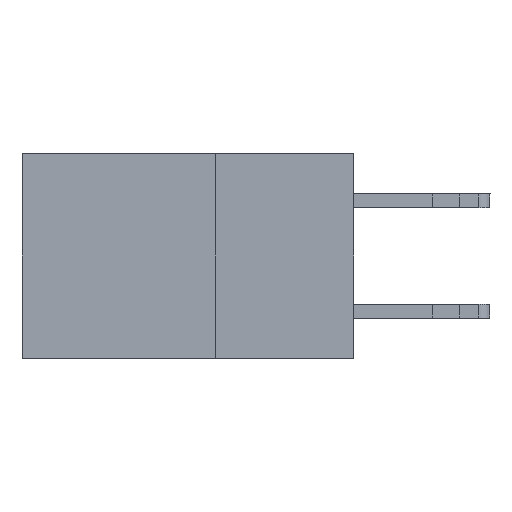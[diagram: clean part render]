
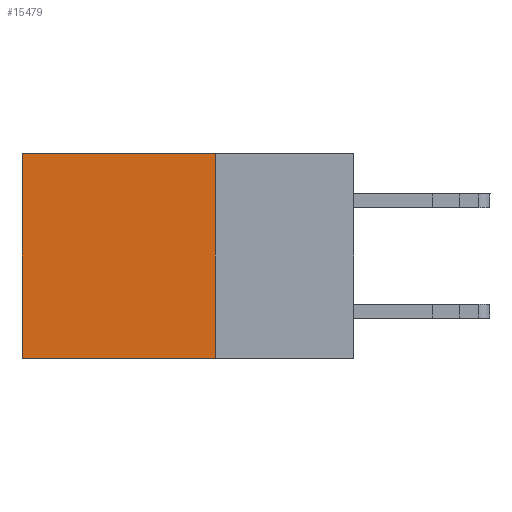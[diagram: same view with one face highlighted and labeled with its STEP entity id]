
A CAD part, left-side view. The second image highlights one B-rep face of the part: STEP entity #15479.
In plain terms, the highlighted planar face has unit normal (-1, 0, 0).
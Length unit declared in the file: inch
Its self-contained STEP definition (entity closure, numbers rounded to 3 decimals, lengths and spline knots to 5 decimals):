
#944 = FACE_OUTER_BOUND ( 'NONE', #14228, .T. ) ;
#1992 = VECTOR ( 'NONE', #2763, 39.37008 ) ;
#2371 = VERTEX_POINT ( 'NONE', #12612 ) ;
#2507 = CARTESIAN_POINT ( 'NONE',  ( 0.2875, 0.25, 0. ) ) ;
#2763 = DIRECTION ( 'NONE',  ( 0., 1., 0. ) ) ;
#3121 = CARTESIAN_POINT ( 'NONE',  ( 0.2875, 0.6, -0.37 ) ) ;
#3181 = VERTEX_POINT ( 'NONE', #2507 ) ;
#4459 = CARTESIAN_POINT ( 'NONE',  ( 0.2875, 0.25, 0. ) ) ;
#5456 = LINE ( 'NONE', #13722, #12056 ) ;
#5554 = LINE ( 'NONE', #9321, #1992 ) ;
#5643 = VERTEX_POINT ( 'NONE', #3121 ) ;
#5786 = DIRECTION ( 'NONE',  ( 0., 1., 0. ) ) ;
#6317 = LINE ( 'NONE', #4459, #16879 ) ;
#6527 = CARTESIAN_POINT ( 'NONE',  ( 0.2875, 0.6, 0. ) ) ;
#7709 = CARTESIAN_POINT ( 'NONE',  ( 0.2875, 0.25, 0. ) ) ;
#7760 = DIRECTION ( 'NONE',  ( 1., 0., 0. ) ) ;
#8071 = EDGE_CURVE ( 'NONE', #9816, #5643, #5456, .T. ) ;
#9321 = CARTESIAN_POINT ( 'NONE',  ( 0.2875, 0.25, -0.37 ) ) ;
#9816 = VERTEX_POINT ( 'NONE', #6527 ) ;
#10898 = ORIENTED_EDGE ( 'NONE', *, *, #8071, .T. ) ;
#12056 = VECTOR ( 'NONE', #15049, 39.37008 ) ;
#12612 = CARTESIAN_POINT ( 'NONE',  ( 0.2875, 0.25, -0.37 ) ) ;
#12794 = CARTESIAN_POINT ( 'NONE',  ( 0.2875, 0.25, 0. ) ) ;
#13560 = EDGE_CURVE ( 'NONE', #3181, #2371, #15769, .T. ) ;
#13722 = CARTESIAN_POINT ( 'NONE',  ( 0.2875, 0.6, 0. ) ) ;
#13879 = ORIENTED_EDGE ( 'NONE', *, *, #16861, .T. ) ;
#14139 = DIRECTION ( 'NONE',  ( 0., 0., -1. ) ) ;
#14228 = EDGE_LOOP ( 'NONE', ( #10898, #16783, #15709, #13879 ) ) ;
#14321 = AXIS2_PLACEMENT_3D ( 'NONE', #7709, #7760, #17016 ) ;
#15049 = DIRECTION ( 'NONE',  ( 0., 0., -1. ) ) ;
#15364 = VECTOR ( 'NONE', #14139, 39.37008 ) ;
#15479 = ADVANCED_FACE ( 'NONE', ( #944 ), #15679, .F. ) ;
#15615 = EDGE_CURVE ( 'NONE', #2371, #5643, #5554, .T. ) ;
#15679 = PLANE ( 'NONE',  #14321 ) ;
#15709 = ORIENTED_EDGE ( 'NONE', *, *, #13560, .F. ) ;
#15769 = LINE ( 'NONE', #12794, #15364 ) ;
#16783 = ORIENTED_EDGE ( 'NONE', *, *, #15615, .F. ) ;
#16861 = EDGE_CURVE ( 'NONE', #3181, #9816, #6317, .T. ) ;
#16879 = VECTOR ( 'NONE', #5786, 39.37008 ) ;
#17016 = DIRECTION ( 'NONE',  ( 0., 0., -1. ) ) ;
